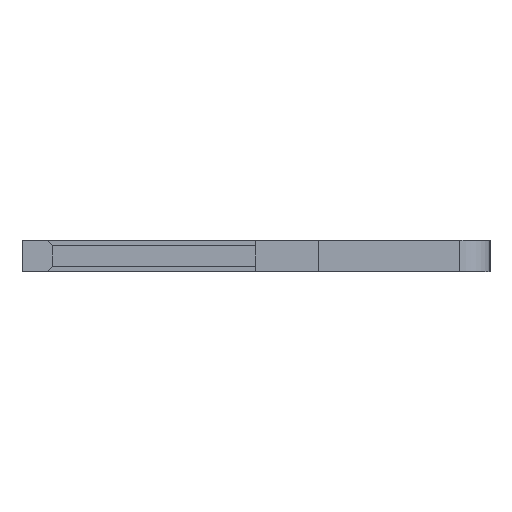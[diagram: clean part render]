
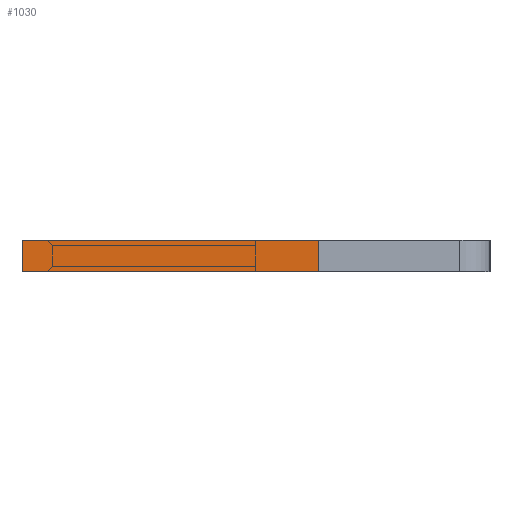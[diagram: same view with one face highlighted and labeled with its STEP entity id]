
A CAD part, left-side view. The second image highlights one B-rep face of the part: STEP entity #1030.
In plain terms, the highlighted face is planar.
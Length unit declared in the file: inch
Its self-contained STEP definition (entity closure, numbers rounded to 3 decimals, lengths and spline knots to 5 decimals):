
#157 = VERTEX_POINT ( 'NONE', #1214 ) ;
#181 = AXIS2_PLACEMENT_3D ( 'NONE', #2212, #2224, #662 ) ;
#205 = DIRECTION ( 'NONE',  ( 0., 1., 0. ) ) ;
#220 = FACE_OUTER_BOUND ( 'NONE', #2753, .T. ) ;
#380 = CARTESIAN_POINT ( 'NONE',  ( -0.01, 0.15, -0.04 ) ) ;
#598 = ORIENTED_EDGE ( 'NONE', *, *, #2848, .F. ) ;
#599 = EDGE_CURVE ( 'NONE', #2913, #647, #3867, .T. ) ;
#647 = VERTEX_POINT ( 'NONE', #3500 ) ;
#662 = DIRECTION ( 'NONE',  ( 1., 0., 0. ) ) ;
#719 = DIRECTION ( 'NONE',  ( -1., 0., 0. ) ) ;
#742 = DIRECTION ( 'NONE',  ( 0., 1., 0. ) ) ;
#793 = ORIENTED_EDGE ( 'NONE', *, *, #1310, .T. ) ;
#1030 = ADVANCED_FACE ( 'NONE', ( #220 ), #1902, .F. ) ;
#1192 = VECTOR ( 'NONE', #205, 39.37008 ) ;
#1214 = CARTESIAN_POINT ( 'NONE',  ( 0.01, 0.15, -0.04 ) ) ;
#1232 = ORIENTED_EDGE ( 'NONE', *, *, #599, .T. ) ;
#1268 = EDGE_CURVE ( 'NONE', #157, #2168, #1350, .T. ) ;
#1276 = CARTESIAN_POINT ( 'NONE',  ( 0.01, -0.04, -0.04 ) ) ;
#1291 = DIRECTION ( 'NONE',  ( -1., 0., 0. ) ) ;
#1310 = EDGE_CURVE ( 'NONE', #647, #2168, #2277, .T. ) ;
#1350 = LINE ( 'NONE', #3854, #1554 ) ;
#1554 = VECTOR ( 'NONE', #719, 39.37008 ) ;
#1848 = VECTOR ( 'NONE', #742, 39.37008 ) ;
#1902 = PLANE ( 'NONE',  #181 ) ;
#2030 = LINE ( 'NONE', #2414, #1192 ) ;
#2168 = VERTEX_POINT ( 'NONE', #3394 ) ;
#2212 = CARTESIAN_POINT ( 'NONE',  ( 0.01, 0.15, -0.04 ) ) ;
#2224 = DIRECTION ( 'NONE',  ( 0., 0., 1. ) ) ;
#2277 = LINE ( 'NONE', #380, #1848 ) ;
#2414 = CARTESIAN_POINT ( 'NONE',  ( 0.01, 0.15, -0.04 ) ) ;
#2753 = EDGE_LOOP ( 'NONE', ( #793, #3495, #598, #1232 ) ) ;
#2848 = EDGE_CURVE ( 'NONE', #2913, #157, #2030, .T. ) ;
#2913 = VERTEX_POINT ( 'NONE', #3667 ) ;
#3049 = VECTOR ( 'NONE', #1291, 39.37008 ) ;
#3394 = CARTESIAN_POINT ( 'NONE',  ( -0.01, 0.15, -0.04 ) ) ;
#3495 = ORIENTED_EDGE ( 'NONE', *, *, #1268, .F. ) ;
#3500 = CARTESIAN_POINT ( 'NONE',  ( -0.01, -0.04, -0.04 ) ) ;
#3667 = CARTESIAN_POINT ( 'NONE',  ( 0.01, -0.04, -0.04 ) ) ;
#3854 = CARTESIAN_POINT ( 'NONE',  ( 0.01, 0.15, -0.04 ) ) ;
#3867 = LINE ( 'NONE', #1276, #3049 ) ;
